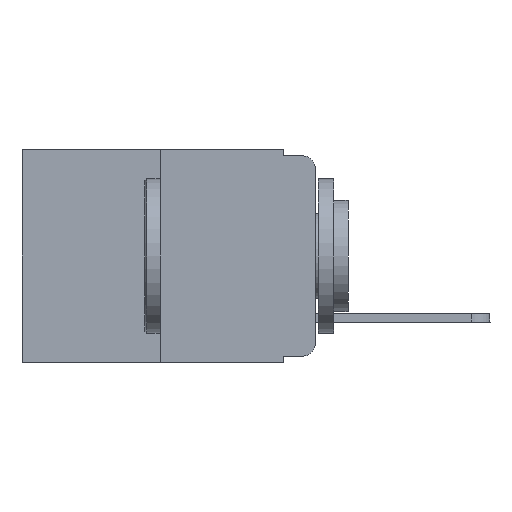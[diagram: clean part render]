
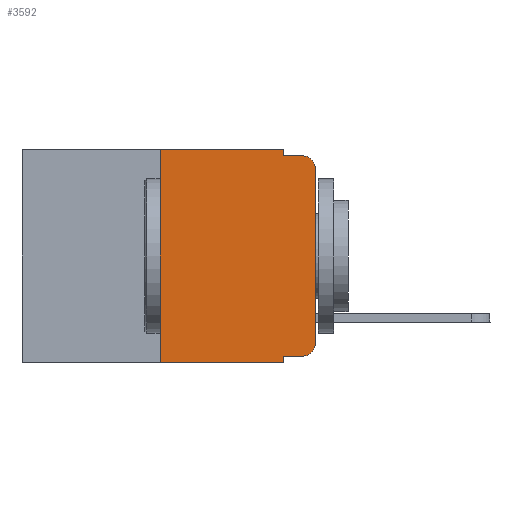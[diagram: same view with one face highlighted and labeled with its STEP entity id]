
A CAD part, left-side view. The second image highlights one B-rep face of the part: STEP entity #3592.
In plain terms, the highlighted planar face has unit normal (-1, 0, 0).
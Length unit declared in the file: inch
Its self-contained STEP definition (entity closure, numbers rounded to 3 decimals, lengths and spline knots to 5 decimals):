
#100 = ORIENTED_EDGE ( 'NONE', *, *, #14747, .T. ) ;
#156 = CARTESIAN_POINT ( 'NONE',  ( 0., 0.25, -0.343 ) ) ;
#294 = EDGE_LOOP ( 'NONE', ( #15364, #100, #18252, #12065, #3881, #12163, #4269, #6904, #9602, #2836 ) ) ;
#395 = CARTESIAN_POINT ( 'NONE',  ( 0., 0.02, -0.313 ) ) ;
#486 = CARTESIAN_POINT ( 'NONE',  ( 0., 0.051, -0.333 ) ) ;
#535 = CIRCLE ( 'NONE', #12051, 0.02 ) ;
#671 = CARTESIAN_POINT ( 'NONE',  ( 0., 0., -0.313 ) ) ;
#1034 = CARTESIAN_POINT ( 'NONE',  ( 0., 0.473, 0. ) ) ;
#1885 = LINE ( 'NONE', #19574, #18547 ) ;
#1927 = CARTESIAN_POINT ( 'NONE',  ( 0., 0.051, 0. ) ) ;
#2204 = EDGE_CURVE ( 'NONE', #4861, #14661, #18591, .T. ) ;
#2537 = DIRECTION ( 'NONE',  ( 0., 0., 1. ) ) ;
#2836 = ORIENTED_EDGE ( 'NONE', *, *, #6165, .T. ) ;
#3412 = VERTEX_POINT ( 'NONE', #486 ) ;
#3479 = CARTESIAN_POINT ( 'NONE',  ( 0., 0.25, 0. ) ) ;
#3592 = ADVANCED_FACE ( 'NONE', ( #17047 ), #4228, .F. ) ;
#3881 = ORIENTED_EDGE ( 'NONE', *, *, #19499, .F. ) ;
#4160 = VECTOR ( 'NONE', #11905, 39.37008 ) ;
#4228 = PLANE ( 'NONE',  #14064 ) ;
#4269 = ORIENTED_EDGE ( 'NONE', *, *, #9109, .T. ) ;
#4294 = DIRECTION ( 'NONE',  ( 1., 0., 0. ) ) ;
#4861 = VERTEX_POINT ( 'NONE', #156 ) ;
#5081 = DIRECTION ( 'NONE',  ( 0., 0., 1. ) ) ;
#5487 = LINE ( 'NONE', #1927, #13029 ) ;
#6005 = CARTESIAN_POINT ( 'NONE',  ( 0., 0., -0.03 ) ) ;
#6165 = EDGE_CURVE ( 'NONE', #7137, #19472, #535, .T. ) ;
#6904 = ORIENTED_EDGE ( 'NONE', *, *, #15473, .F. ) ;
#7000 = EDGE_CURVE ( 'NONE', #12906, #16858, #5487, .T. ) ;
#7032 = VECTOR ( 'NONE', #11040, 39.37008 ) ;
#7137 = VERTEX_POINT ( 'NONE', #7828 ) ;
#7422 = CARTESIAN_POINT ( 'NONE',  ( 0., 0.051, -0.01 ) ) ;
#7828 = CARTESIAN_POINT ( 'NONE',  ( 0., 0.02, -0.333 ) ) ;
#7884 = CARTESIAN_POINT ( 'NONE',  ( 0., 0.051, -0.01 ) ) ;
#8052 = VECTOR ( 'NONE', #17299, 39.37008 ) ;
#8326 = VECTOR ( 'NONE', #19160, 39.37008 ) ;
#8429 = EDGE_CURVE ( 'NONE', #19472, #18927, #1885, .T. ) ;
#8581 = DIRECTION ( 'NONE',  ( 0., -1., 0. ) ) ;
#8640 = DIRECTION ( 'NONE',  ( 0., 0., -1. ) ) ;
#8810 = VERTEX_POINT ( 'NONE', #11686 ) ;
#8859 = CARTESIAN_POINT ( 'NONE',  ( 0., 0.25, 0. ) ) ;
#9072 = DIRECTION ( 'NONE',  ( -1., 0., 0. ) ) ;
#9109 = EDGE_CURVE ( 'NONE', #4861, #8810, #11378, .T. ) ;
#9602 = ORIENTED_EDGE ( 'NONE', *, *, #11168, .T. ) ;
#10279 = CARTESIAN_POINT ( 'NONE',  ( 0., 0.473, -0.343 ) ) ;
#10554 = LINE ( 'NONE', #14169, #7032 ) ;
#10589 = CARTESIAN_POINT ( 'NONE',  ( 0., 0.02, -0.01 ) ) ;
#11040 = DIRECTION ( 'NONE',  ( 0., -1., 0. ) ) ;
#11168 = EDGE_CURVE ( 'NONE', #3412, #7137, #10554, .T. ) ;
#11184 = VECTOR ( 'NONE', #8581, 39.37008 ) ;
#11378 = LINE ( 'NONE', #10279, #4160 ) ;
#11686 = CARTESIAN_POINT ( 'NONE',  ( 0., 0.051, -0.343 ) ) ;
#11905 = DIRECTION ( 'NONE',  ( 0., -1., 0. ) ) ;
#12051 = AXIS2_PLACEMENT_3D ( 'NONE', #395, #14946, #8640 ) ;
#12065 = ORIENTED_EDGE ( 'NONE', *, *, #7000, .F. ) ;
#12121 = CARTESIAN_POINT ( 'NONE',  ( 0., 0.02, -0.03 ) ) ;
#12163 = ORIENTED_EDGE ( 'NONE', *, *, #2204, .F. ) ;
#12906 = VERTEX_POINT ( 'NONE', #19604 ) ;
#13029 = VECTOR ( 'NONE', #15514, 39.37008 ) ;
#13357 = LINE ( 'NONE', #15492, #8052 ) ;
#14064 = AXIS2_PLACEMENT_3D ( 'NONE', #1034, #4294, #15534 ) ;
#14169 = CARTESIAN_POINT ( 'NONE',  ( 0., 0.051, -0.333 ) ) ;
#14256 = VECTOR ( 'NONE', #5081, 39.37008 ) ;
#14661 = VERTEX_POINT ( 'NONE', #8859 ) ;
#14747 = EDGE_CURVE ( 'NONE', #18927, #20700, #17998, .T. ) ;
#14843 = EDGE_CURVE ( 'NONE', #16858, #20700, #18498, .T. ) ;
#14946 = DIRECTION ( 'NONE',  ( -1., 0., 0. ) ) ;
#15013 = CARTESIAN_POINT ( 'NONE',  ( 0., 0.473, 0. ) ) ;
#15364 = ORIENTED_EDGE ( 'NONE', *, *, #8429, .T. ) ;
#15451 = DIRECTION ( 'NONE',  ( 0., 0., -1. ) ) ;
#15473 = EDGE_CURVE ( 'NONE', #3412, #8810, #13357, .T. ) ;
#15492 = CARTESIAN_POINT ( 'NONE',  ( 0., 0.051, 0. ) ) ;
#15514 = DIRECTION ( 'NONE',  ( 0., 0., -1. ) ) ;
#15534 = DIRECTION ( 'NONE',  ( 0., 0., -1. ) ) ;
#16858 = VERTEX_POINT ( 'NONE', #7422 ) ;
#17047 = FACE_OUTER_BOUND ( 'NONE', #294, .T. ) ;
#17299 = DIRECTION ( 'NONE',  ( 0., 0., -1. ) ) ;
#17998 = CIRCLE ( 'NONE', #18698, 0.02 ) ;
#18252 = ORIENTED_EDGE ( 'NONE', *, *, #14843, .F. ) ;
#18498 = LINE ( 'NONE', #7884, #8326 ) ;
#18547 = VECTOR ( 'NONE', #2537, 39.37008 ) ;
#18591 = LINE ( 'NONE', #3479, #14256 ) ;
#18698 = AXIS2_PLACEMENT_3D ( 'NONE', #12121, #9072, #15451 ) ;
#18927 = VERTEX_POINT ( 'NONE', #6005 ) ;
#19160 = DIRECTION ( 'NONE',  ( 0., -1., 0. ) ) ;
#19472 = VERTEX_POINT ( 'NONE', #671 ) ;
#19499 = EDGE_CURVE ( 'NONE', #14661, #12906, #20338, .T. ) ;
#19574 = CARTESIAN_POINT ( 'NONE',  ( 0., 0., 0. ) ) ;
#19604 = CARTESIAN_POINT ( 'NONE',  ( 0., 0.051, 0. ) ) ;
#20338 = LINE ( 'NONE', #15013, #11184 ) ;
#20700 = VERTEX_POINT ( 'NONE', #10589 ) ;
